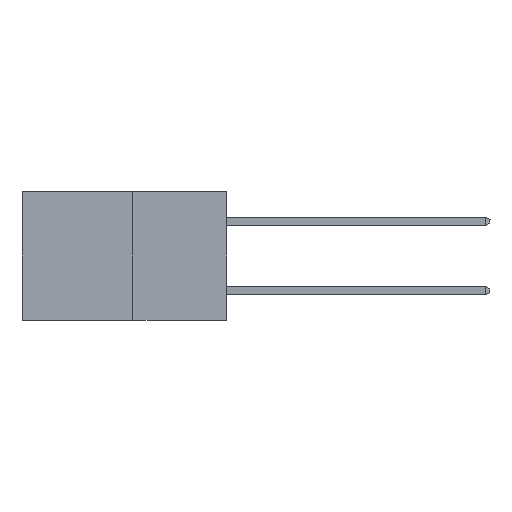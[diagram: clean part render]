
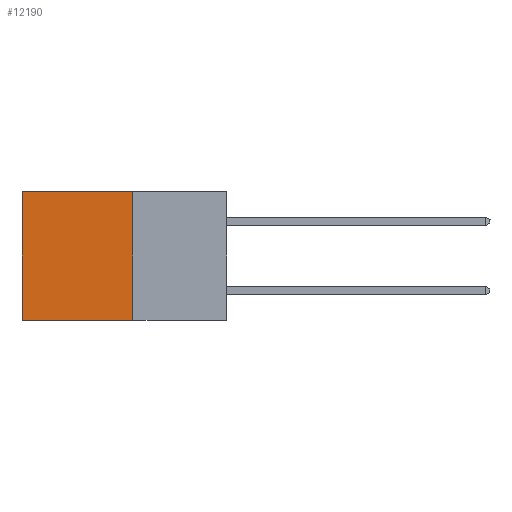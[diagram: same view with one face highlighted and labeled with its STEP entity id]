
A CAD part, left-side view. The second image highlights one B-rep face of the part: STEP entity #12190.
In plain terms, the highlighted planar face has unit normal (-1, 0, 0).
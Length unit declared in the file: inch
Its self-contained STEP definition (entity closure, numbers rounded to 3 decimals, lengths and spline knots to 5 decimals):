
#1391 = CARTESIAN_POINT ( 'NONE',  ( 0.277, 0.59, 0. ) ) ;
#1425 = CARTESIAN_POINT ( 'NONE',  ( 0.277, 0.59, -0.37 ) ) ;
#1550 = EDGE_CURVE ( 'NONE', #18947, #2023, #5711, .T. ) ;
#1856 = VERTEX_POINT ( 'NONE', #11661 ) ;
#2023 = VERTEX_POINT ( 'NONE', #1391 ) ;
#2402 = ORIENTED_EDGE ( 'NONE', *, *, #6254, .F. ) ;
#2816 = DIRECTION ( 'NONE',  ( 0., 0., -1. ) ) ;
#2856 = ORIENTED_EDGE ( 'NONE', *, *, #1550, .T. ) ;
#3345 = DIRECTION ( 'NONE',  ( 1., 0., 0. ) ) ;
#4650 = LINE ( 'NONE', #16051, #12516 ) ;
#4890 = LINE ( 'NONE', #1425, #13220 ) ;
#5457 = AXIS2_PLACEMENT_3D ( 'NONE', #15196, #3345, #13754 ) ;
#5711 = LINE ( 'NONE', #9827, #9213 ) ;
#6207 = CARTESIAN_POINT ( 'NONE',  ( 0.277, 0.27, 0. ) ) ;
#6254 = EDGE_CURVE ( 'NONE', #18947, #19255, #9973, .T. ) ;
#8309 = CARTESIAN_POINT ( 'NONE',  ( 0.277, 0.27, -0.37 ) ) ;
#8392 = DIRECTION ( 'NONE',  ( 0., 0., -1. ) ) ;
#8464 = EDGE_LOOP ( 'NONE', ( #15202, #18004, #2402, #2856 ) ) ;
#9213 = VECTOR ( 'NONE', #10244, 39.37008 ) ;
#9332 = PLANE ( 'NONE',  #5457 ) ;
#9529 = VECTOR ( 'NONE', #8392, 39.37008 ) ;
#9827 = CARTESIAN_POINT ( 'NONE',  ( 0.277, 0.27, 0. ) ) ;
#9973 = LINE ( 'NONE', #8309, #9529 ) ;
#10244 = DIRECTION ( 'NONE',  ( 0., 1., 0. ) ) ;
#10954 = EDGE_CURVE ( 'NONE', #2023, #1856, #4890, .T. ) ;
#11661 = CARTESIAN_POINT ( 'NONE',  ( 0.277, 0.59, -0.37 ) ) ;
#11895 = EDGE_CURVE ( 'NONE', #19255, #1856, #4650, .T. ) ;
#12190 = ADVANCED_FACE ( 'NONE', ( #18855 ), #9332, .F. ) ;
#12516 = VECTOR ( 'NONE', #17554, 39.37008 ) ;
#13220 = VECTOR ( 'NONE', #2816, 39.37008 ) ;
#13754 = DIRECTION ( 'NONE',  ( 0., 0., -1. ) ) ;
#14184 = CARTESIAN_POINT ( 'NONE',  ( 0.277, 0.27, -0.37 ) ) ;
#15196 = CARTESIAN_POINT ( 'NONE',  ( 0.277, 0.27, -0.37 ) ) ;
#15202 = ORIENTED_EDGE ( 'NONE', *, *, #10954, .T. ) ;
#16051 = CARTESIAN_POINT ( 'NONE',  ( 0.277, 0.27, -0.37 ) ) ;
#17554 = DIRECTION ( 'NONE',  ( 0., 1., 0. ) ) ;
#18004 = ORIENTED_EDGE ( 'NONE', *, *, #11895, .F. ) ;
#18855 = FACE_OUTER_BOUND ( 'NONE', #8464, .T. ) ;
#18947 = VERTEX_POINT ( 'NONE', #6207 ) ;
#19255 = VERTEX_POINT ( 'NONE', #14184 ) ;
